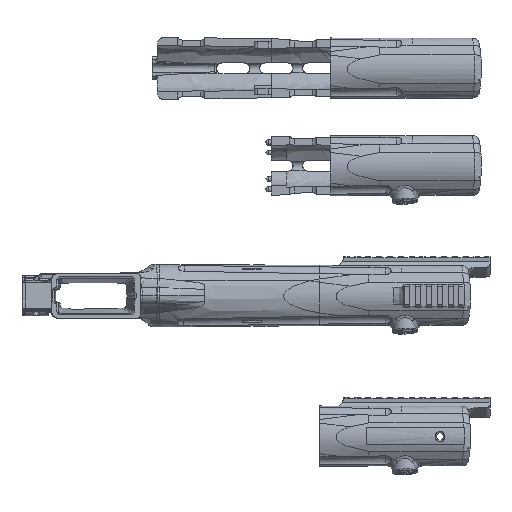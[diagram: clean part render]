
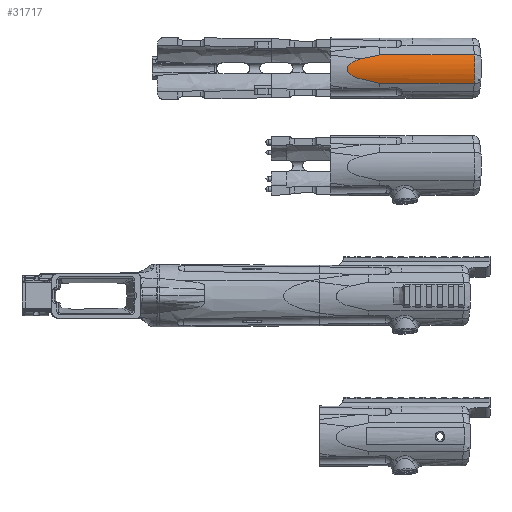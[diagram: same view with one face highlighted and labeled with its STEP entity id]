
A CAD part, front view. The second image highlights one B-rep face of the part: STEP entity #31717.
In plain terms, the highlighted cylindrical face has radius 29.942 mm (diameter 59.884 mm), a partial arc.
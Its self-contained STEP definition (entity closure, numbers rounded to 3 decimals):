
#64=ELLIPSE('',#33691,30.258,29.942);
#2224=B_SPLINE_CURVE_WITH_KNOTS('',3,(#69375,#69376,#69377,#69378),
 .UNSPECIFIED.,.F.,.F.,(4,4),(-22.321,-11.02),
 .UNSPECIFIED.);
#2285=B_SPLINE_CURVE_WITH_KNOTS('',3,(#70509,#70510,#70511,#70512,#70513,
#70514,#70515,#70516,#70517,#70518,#70519,#70520,#70521,#70522,#70523,#70524,
#70525,#70526,#70527,#70528,#70529,#70530),.UNSPECIFIED.,.F.,.F.,(4,1,1,
1,1,1,1,1,2,1,1,1,1,1,1,1,1,1,4),(-67.905,-66.347,-57.432,
-55.203,-54.088,-53.531,-53.253,
-53.113,-52.974,-51.65,-50.325,
-47.677,-42.379,-31.784,-21.19,
-10.595,-5.297,-2.649,0.),
 .UNSPECIFIED.);
#4899=FACE_OUTER_BOUND('',#6734,.T.);
#6734=EDGE_LOOP('',(#28450,#28451,#28452,#28453,#28454));
#9093=LINE('',#70499,#11363);
#9094=LINE('',#70508,#11364);
#11363=VECTOR('',#39418,10.);
#11364=VECTOR('',#39421,10.);
#14896=VERTEX_POINT('',#69372);
#14897=VERTEX_POINT('',#69374);
#14937=VERTEX_POINT('',#70149);
#14942=VERTEX_POINT('',#70204);
#14955=VERTEX_POINT('',#70498);
#19469=EDGE_CURVE('',#14896,#14897,#2224,.T.);
#19528=EDGE_CURVE('',#14942,#14937,#64,.T.);
#19546=EDGE_CURVE('',#14955,#14937,#9093,.T.);
#19548=EDGE_CURVE('',#14897,#14942,#9094,.T.);
#19549=EDGE_CURVE('',#14955,#14896,#2285,.T.);
#28450=ORIENTED_EDGE('',*,*,#19528,.F.);
#28451=ORIENTED_EDGE('',*,*,#19548,.F.);
#28452=ORIENTED_EDGE('',*,*,#19469,.F.);
#28453=ORIENTED_EDGE('',*,*,#19549,.F.);
#28454=ORIENTED_EDGE('',*,*,#19546,.T.);
#30177=CYLINDRICAL_SURFACE('',#33693,29.942);
#31717=ADVANCED_FACE('',(#4899),#30177,.T.);
#33691=AXIS2_PLACEMENT_3D('',#70206,#39413,#39414);
#33693=AXIS2_PLACEMENT_3D('',#70507,#39419,#39420);
#39413=DIRECTION('center_axis',(0.99,0.144,0.));
#39414=DIRECTION('ref_axis',(0.144,-0.99,0.));
#39418=DIRECTION('',(1.,0.,0.));
#39419=DIRECTION('center_axis',(-1.,0.,0.));
#39420=DIRECTION('ref_axis',(0.,-1.,-0.024));
#39421=DIRECTION('',(1.,0.,0.));
#69372=CARTESIAN_POINT('',(198.362,-6.262,218.824));
#69374=CARTESIAN_POINT('',(215.42,-4.887,222.411));
#69375=CARTESIAN_POINT('Ctrl Pts',(198.362,-6.262,218.824));
#69376=CARTESIAN_POINT('Ctrl Pts',(203.153,-5.88,220.052));
#69377=CARTESIAN_POINT('Ctrl Pts',(208.685,-5.418,221.252));
#69378=CARTESIAN_POINT('Ctrl Pts',(215.42,-4.886,222.412));
#70149=CARTESIAN_POINT('',(302.809,-4.265,196.162));
#70204=CARTESIAN_POINT('',(302.9,-4.887,222.411));
#70206=CARTESIAN_POINT('Origin',(298.935,22.327,209.924));
#70498=CARTESIAN_POINT('',(215.42,-4.265,196.162));
#70499=CARTESIAN_POINT('',(215.42,-4.265,196.162));
#70507=CARTESIAN_POINT('Origin',(215.42,22.327,209.924));
#70508=CARTESIAN_POINT('',(215.42,-4.887,222.411));
#70509=CARTESIAN_POINT('Ctrl Pts',(215.42,-4.265,196.162));
#70510=CARTESIAN_POINT('Ctrl Pts',(214.577,-4.347,196.32));
#70511=CARTESIAN_POINT('Ctrl Pts',(209.026,-4.885,197.383));
#70512=CARTESIAN_POINT('Ctrl Pts',(203.242,-5.464,198.718));
#70513=CARTESIAN_POINT('Ctrl Pts',(198.415,-5.938,200.037));
#70514=CARTESIAN_POINT('Ctrl Pts',(196.945,-6.08,200.459));
#70515=CARTESIAN_POINT('Ctrl Pts',(196.226,-6.15,200.671));
#70516=CARTESIAN_POINT('Ctrl Pts',(195.87,-6.184,200.777));
#70517=CARTESIAN_POINT('Ctrl Pts',(195.668,-6.203,200.837));
#70518=CARTESIAN_POINT('Ctrl Pts',(195.567,-6.213,200.868));
#70519=CARTESIAN_POINT('Ctrl Pts',(195.039,-6.263,201.027));
#70520=CARTESIAN_POINT('Ctrl Pts',(194.144,-6.353,201.316));
#70521=CARTESIAN_POINT('Ctrl Pts',(192.563,-6.522,201.897));
#70522=CARTESIAN_POINT('Ctrl Pts',(190.246,-6.796,202.923));
#70523=CARTESIAN_POINT('Ctrl Pts',(187.055,-7.252,205.003));
#70524=CARTESIAN_POINT('Ctrl Pts',(185.11,-7.629,208.024));
#70525=CARTESIAN_POINT('Ctrl Pts',(185.525,-7.638,211.679));
#70526=CARTESIAN_POINT('Ctrl Pts',(188.227,-7.275,214.701));
#70527=CARTESIAN_POINT('Ctrl Pts',(192.121,-6.83,216.783));
#70528=CARTESIAN_POINT('Ctrl Pts',(195.271,-6.522,217.956));
#70529=CARTESIAN_POINT('Ctrl Pts',(197.239,-6.351,218.536));
#70530=CARTESIAN_POINT('Ctrl Pts',(198.362,-6.262,218.824));
